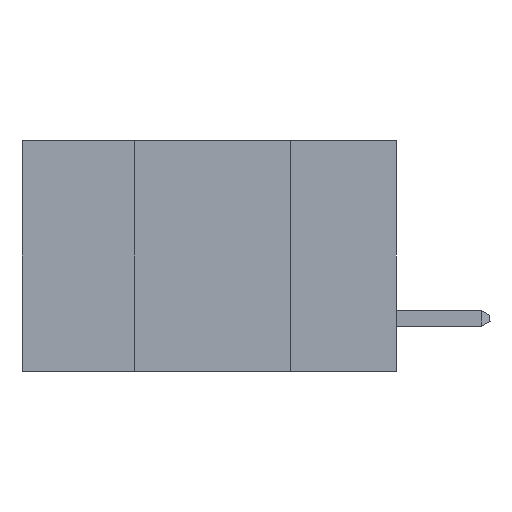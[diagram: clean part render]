
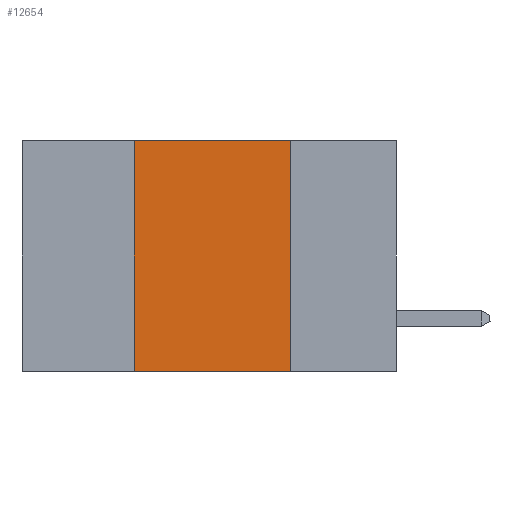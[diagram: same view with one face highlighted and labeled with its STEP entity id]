
A CAD part, left-side view. The second image highlights one B-rep face of the part: STEP entity #12654.
In plain terms, the highlighted planar face has unit normal (-1, 0, 0).
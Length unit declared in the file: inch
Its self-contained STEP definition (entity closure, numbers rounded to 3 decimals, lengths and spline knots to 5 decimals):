
#40 = EDGE_CURVE ( 'NONE', #4287, #3393, #5489, .T. ) ;
#87 = CARTESIAN_POINT ( 'NONE',  ( 0., 0.17, 0. ) ) ;
#455 = EDGE_CURVE ( 'NONE', #1567, #3499, #3128, .T. ) ;
#1258 = ORIENTED_EDGE ( 'NONE', *, *, #455, .F. ) ;
#1567 = VERTEX_POINT ( 'NONE', #7530 ) ;
#1857 = VECTOR ( 'NONE', #9195, 39.37008 ) ;
#3128 = LINE ( 'NONE', #6152, #1857 ) ;
#3136 = LINE ( 'NONE', #6571, #4577 ) ;
#3150 = DIRECTION ( 'NONE',  ( 0., -1., 0. ) ) ;
#3393 = VERTEX_POINT ( 'NONE', #5115 ) ;
#3499 = VERTEX_POINT ( 'NONE', #11708 ) ;
#4148 = LINE ( 'NONE', #11600, #8862 ) ;
#4287 = VERTEX_POINT ( 'NONE', #87 ) ;
#4577 = VECTOR ( 'NONE', #8568, 39.37008 ) ;
#4701 = EDGE_CURVE ( 'NONE', #1567, #3393, #4148, .T. ) ;
#5115 = CARTESIAN_POINT ( 'NONE',  ( 0., 0.17, -0.37 ) ) ;
#5220 = CARTESIAN_POINT ( 'NONE',  ( 0., 0.6, 0. ) ) ;
#5489 = LINE ( 'NONE', #10501, #8184 ) ;
#6152 = CARTESIAN_POINT ( 'NONE',  ( 0., 0.42, 0. ) ) ;
#6334 = FACE_OUTER_BOUND ( 'NONE', #10521, .T. ) ;
#6571 = CARTESIAN_POINT ( 'NONE',  ( 0., 0.6, 0. ) ) ;
#7499 = ORIENTED_EDGE ( 'NONE', *, *, #40, .F. ) ;
#7530 = CARTESIAN_POINT ( 'NONE',  ( 0., 0.42, -0.37 ) ) ;
#8085 = PLANE ( 'NONE',  #9580 ) ;
#8184 = VECTOR ( 'NONE', #10541, 39.37008 ) ;
#8487 = EDGE_CURVE ( 'NONE', #3499, #4287, #3136, .T. ) ;
#8568 = DIRECTION ( 'NONE',  ( 0., -1., 0. ) ) ;
#8862 = VECTOR ( 'NONE', #3150, 39.37008 ) ;
#8935 = ORIENTED_EDGE ( 'NONE', *, *, #4701, .T. ) ;
#9170 = DIRECTION ( 'NONE',  ( 1., 0., 0. ) ) ;
#9195 = DIRECTION ( 'NONE',  ( 0., 0., 1. ) ) ;
#9580 = AXIS2_PLACEMENT_3D ( 'NONE', #5220, #9170, #11222 ) ;
#10501 = CARTESIAN_POINT ( 'NONE',  ( 0., 0.17, 0. ) ) ;
#10521 = EDGE_LOOP ( 'NONE', ( #7499, #12716, #1258, #8935 ) ) ;
#10541 = DIRECTION ( 'NONE',  ( 0., 0., -1. ) ) ;
#11222 = DIRECTION ( 'NONE',  ( 0., 0., -1. ) ) ;
#11600 = CARTESIAN_POINT ( 'NONE',  ( 0., 0.6, -0.37 ) ) ;
#11708 = CARTESIAN_POINT ( 'NONE',  ( 0., 0.42, 0. ) ) ;
#12654 = ADVANCED_FACE ( 'NONE', ( #6334 ), #8085, .F. ) ;
#12716 = ORIENTED_EDGE ( 'NONE', *, *, #8487, .F. ) ;
